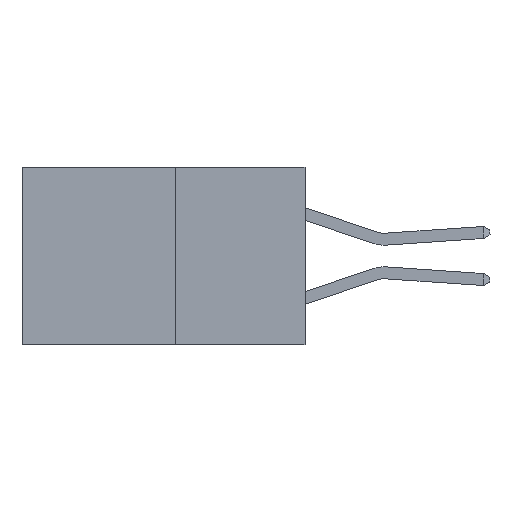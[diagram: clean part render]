
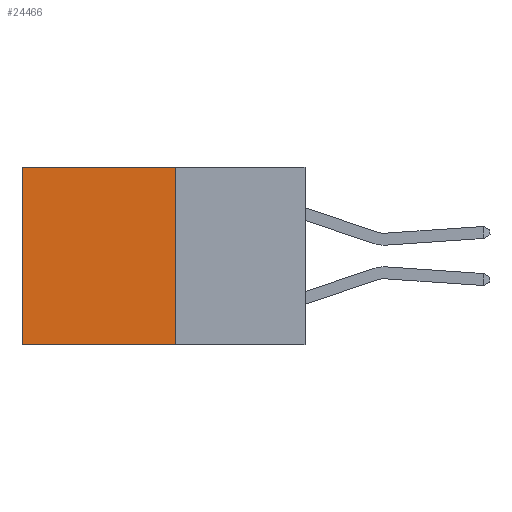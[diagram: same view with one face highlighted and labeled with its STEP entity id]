
A CAD part, left-side view. The second image highlights one B-rep face of the part: STEP entity #24466.
In plain terms, the highlighted planar face has unit normal (-1, 0, 0).
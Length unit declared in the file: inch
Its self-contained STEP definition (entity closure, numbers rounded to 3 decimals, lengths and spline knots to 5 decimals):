
#689 = CARTESIAN_POINT ( 'NONE',  ( 0.277, 0.59, -0.37 ) ) ;
#806 = VERTEX_POINT ( 'NONE', #12767 ) ;
#985 = VECTOR ( 'NONE', #21952, 39.37008 ) ;
#1601 = LINE ( 'NONE', #10378, #985 ) ;
#2355 = LINE ( 'NONE', #689, #12165 ) ;
#2640 = DIRECTION ( 'NONE',  ( 0., 0., -1. ) ) ;
#3332 = VERTEX_POINT ( 'NONE', #10854 ) ;
#4908 = VECTOR ( 'NONE', #12325, 39.37008 ) ;
#7383 = LINE ( 'NONE', #20410, #24567 ) ;
#8486 = EDGE_CURVE ( 'NONE', #3332, #11039, #2355, .T. ) ;
#8528 = CARTESIAN_POINT ( 'NONE',  ( 0.277, 0.27, 0. ) ) ;
#8896 = DIRECTION ( 'NONE',  ( 0., 0., -1. ) ) ;
#9749 = PLANE ( 'NONE',  #19621 ) ;
#10378 = CARTESIAN_POINT ( 'NONE',  ( 0.277, 0.27, -0.37 ) ) ;
#10506 = CARTESIAN_POINT ( 'NONE',  ( 0.277, 0.59, -0.37 ) ) ;
#10854 = CARTESIAN_POINT ( 'NONE',  ( 0.277, 0.59, 0. ) ) ;
#11039 = VERTEX_POINT ( 'NONE', #10506 ) ;
#11108 = EDGE_LOOP ( 'NONE', ( #12688, #24605, #15213, #25055 ) ) ;
#12165 = VECTOR ( 'NONE', #2640, 39.37008 ) ;
#12325 = DIRECTION ( 'NONE',  ( 0., 1., 0. ) ) ;
#12688 = ORIENTED_EDGE ( 'NONE', *, *, #8486, .T. ) ;
#12767 = CARTESIAN_POINT ( 'NONE',  ( 0.277, 0.27, -0.37 ) ) ;
#13632 = DIRECTION ( 'NONE',  ( 0., 0., -1. ) ) ;
#13811 = EDGE_CURVE ( 'NONE', #14213, #806, #7383, .T. ) ;
#14213 = VERTEX_POINT ( 'NONE', #15648 ) ;
#15213 = ORIENTED_EDGE ( 'NONE', *, *, #13811, .F. ) ;
#15479 = CARTESIAN_POINT ( 'NONE',  ( 0.277, 0.27, -0.37 ) ) ;
#15648 = CARTESIAN_POINT ( 'NONE',  ( 0.277, 0.27, 0. ) ) ;
#15837 = LINE ( 'NONE', #8528, #4908 ) ;
#18453 = DIRECTION ( 'NONE',  ( 1., 0., 0. ) ) ;
#18748 = EDGE_CURVE ( 'NONE', #806, #11039, #1601, .T. ) ;
#19621 = AXIS2_PLACEMENT_3D ( 'NONE', #15479, #18453, #13632 ) ;
#20410 = CARTESIAN_POINT ( 'NONE',  ( 0.277, 0.27, -0.37 ) ) ;
#20547 = FACE_OUTER_BOUND ( 'NONE', #11108, .T. ) ;
#21952 = DIRECTION ( 'NONE',  ( 0., 1., 0. ) ) ;
#23304 = EDGE_CURVE ( 'NONE', #14213, #3332, #15837, .T. ) ;
#24466 = ADVANCED_FACE ( 'NONE', ( #20547 ), #9749, .F. ) ;
#24567 = VECTOR ( 'NONE', #8896, 39.37008 ) ;
#24605 = ORIENTED_EDGE ( 'NONE', *, *, #18748, .F. ) ;
#25055 = ORIENTED_EDGE ( 'NONE', *, *, #23304, .T. ) ;
